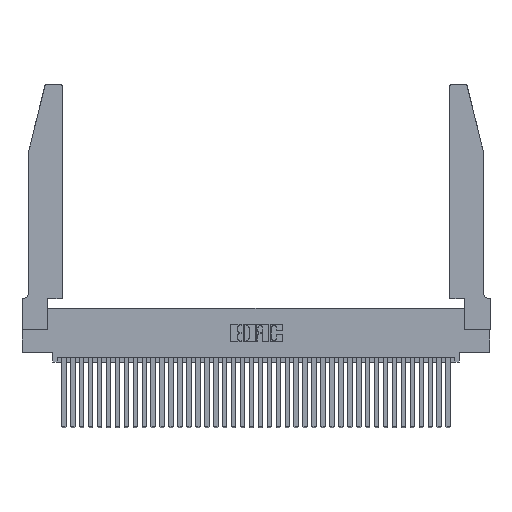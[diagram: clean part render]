
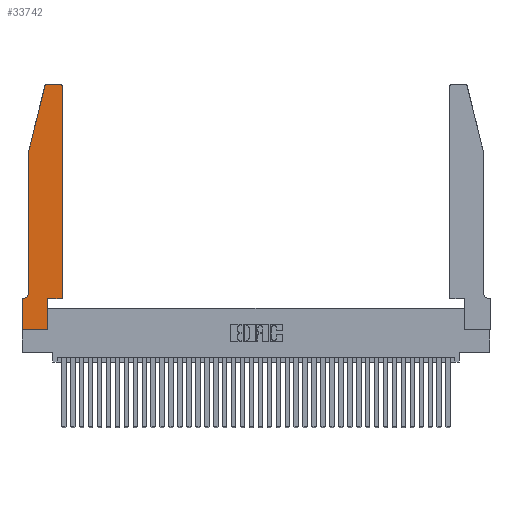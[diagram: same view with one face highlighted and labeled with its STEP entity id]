
A CAD part, top view. The second image highlights one B-rep face of the part: STEP entity #33742.
In plain terms, the highlighted planar face has unit normal (0, 0, 1).
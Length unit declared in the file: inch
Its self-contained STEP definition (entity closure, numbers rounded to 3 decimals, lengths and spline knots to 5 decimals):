
#1102 = EDGE_CURVE ( 'NONE', #10972, #13277, #33385, .T. ) ;
#1503 = VERTEX_POINT ( 'NONE', #20617 ) ;
#1673 = CARTESIAN_POINT ( 'NONE',  ( 0.0755, 2., 0.37 ) ) ;
#1690 = DIRECTION ( 'NONE',  ( 1., 0., 0. ) ) ;
#2762 = DIRECTION ( 'NONE',  ( 0., -1., 0. ) ) ;
#3133 = DIRECTION ( 'NONE',  ( 1., 0., 0. ) ) ;
#3369 = LINE ( 'NONE', #26260, #16984 ) ;
#3413 = LINE ( 'NONE', #1673, #31639 ) ;
#3737 = ORIENTED_EDGE ( 'NONE', *, *, #11222, .T. ) ;
#3932 = ORIENTED_EDGE ( 'NONE', *, *, #10514, .T. ) ;
#5132 = ORIENTED_EDGE ( 'NONE', *, *, #38542, .T. ) ;
#5758 = AXIS2_PLACEMENT_3D ( 'NONE', #37495, #10068, #19400 ) ;
#5767 = CARTESIAN_POINT ( 'NONE',  ( 0.4505, 0.35, 0.37 ) ) ;
#5779 = DIRECTION ( 'NONE',  ( 1., 0., 0. ) ) ;
#6118 = VERTEX_POINT ( 'NONE', #27946 ) ;
#7369 = CARTESIAN_POINT ( 'NONE',  ( 0.0755, 2., 0.37 ) ) ;
#7943 = ORIENTED_EDGE ( 'NONE', *, *, #11675, .T. ) ;
#8167 = EDGE_CURVE ( 'NONE', #6118, #37233, #38728, .T. ) ;
#8539 = CARTESIAN_POINT ( 'NONE',  ( 0., 0., 0.37 ) ) ;
#9168 = VECTOR ( 'NONE', #2762, 39.37008 ) ;
#9340 = AXIS2_PLACEMENT_3D ( 'NONE', #27116, #26991, #33083 ) ;
#9657 = DIRECTION ( 'NONE',  ( 0., 1., 0. ) ) ;
#10068 = DIRECTION ( 'NONE',  ( 0., 0., -1. ) ) ;
#10113 = ORIENTED_EDGE ( 'NONE', *, *, #28743, .T. ) ;
#10354 = VECTOR ( 'NONE', #3133, 39.37008 ) ;
#10514 = EDGE_CURVE ( 'NONE', #37233, #19504, #33564, .T. ) ;
#10587 = VERTEX_POINT ( 'NONE', #28307 ) ;
#10622 = CARTESIAN_POINT ( 'NONE',  ( 0.284, 2.72, 0.37 ) ) ;
#10972 = VERTEX_POINT ( 'NONE', #17748 ) ;
#11222 = EDGE_CURVE ( 'NONE', #36231, #1503, #25538, .T. ) ;
#11424 = PLANE ( 'NONE',  #25909 ) ;
#11675 = EDGE_CURVE ( 'NONE', #10587, #27237, #3369, .T. ) ;
#12286 = CARTESIAN_POINT ( 'NONE',  ( 0.0055, 0.35, 0.37 ) ) ;
#13109 = CARTESIAN_POINT ( 'NONE',  ( 0.0755, 0.35, 0.37 ) ) ;
#13259 = LINE ( 'NONE', #21642, #21733 ) ;
#13277 = VERTEX_POINT ( 'NONE', #37921 ) ;
#13508 = CIRCLE ( 'NONE', #5758, 0.07 ) ;
#13902 = EDGE_CURVE ( 'NONE', #13277, #36231, #13508, .T. ) ;
#15530 = ORIENTED_EDGE ( 'NONE', *, *, #8167, .T. ) ;
#16342 = DIRECTION ( 'NONE',  ( 1., 0., 0. ) ) ;
#16609 = DIRECTION ( 'NONE',  ( 0., 0., 1. ) ) ;
#16892 = ORIENTED_EDGE ( 'NONE', *, *, #26562, .T. ) ;
#16984 = VECTOR ( 'NONE', #26904, 39.37008 ) ;
#17439 = VECTOR ( 'NONE', #16342, 39.37008 ) ;
#17500 = VECTOR ( 'NONE', #9657, 39.37008 ) ;
#17505 = VECTOR ( 'NONE', #18923, 39.37008 ) ;
#17748 = CARTESIAN_POINT ( 'NONE',  ( 0.0755, 2., 0.37 ) ) ;
#18323 = LINE ( 'NONE', #5767, #10354 ) ;
#18704 = AXIS2_PLACEMENT_3D ( 'NONE', #10622, #16609, #1690 ) ;
#18923 = DIRECTION ( 'NONE',  ( -1., 0., 0. ) ) ;
#19398 = DIRECTION ( 'NONE',  ( -0.239, -0.971, 0. ) ) ;
#19400 = DIRECTION ( 'NONE',  ( -1., 0., 0. ) ) ;
#19466 = ORIENTED_EDGE ( 'NONE', *, *, #1102, .T. ) ;
#19504 = VERTEX_POINT ( 'NONE', #29045 ) ;
#19529 = CARTESIAN_POINT ( 'NONE',  ( 0., 0., 0.37 ) ) ;
#20617 = CARTESIAN_POINT ( 'NONE',  ( 0., 0.35, 0.37 ) ) ;
#20677 = EDGE_CURVE ( 'NONE', #27237, #36382, #22739, .T. ) ;
#21576 = EDGE_LOOP ( 'NONE', ( #7943, #35192, #33126, #19466, #24120, #3737, #33429, #15530, #3932, #16892, #10113, #5132 ) ) ;
#21642 = CARTESIAN_POINT ( 'NONE',  ( 0.4505, 0.35, 0.37 ) ) ;
#21733 = VECTOR ( 'NONE', #30726, 39.37008 ) ;
#22739 = CIRCLE ( 'NONE', #18704, 0.03 ) ;
#23288 = CARTESIAN_POINT ( 'NONE',  ( 0.2865, 0., 0.37 ) ) ;
#23658 = CARTESIAN_POINT ( 'NONE',  ( 0., 0.35, 0.37 ) ) ;
#24016 = CIRCLE ( 'NONE', #9340, 0.03 ) ;
#24120 = ORIENTED_EDGE ( 'NONE', *, *, #13902, .T. ) ;
#24608 = VERTEX_POINT ( 'NONE', #25740 ) ;
#24628 = CARTESIAN_POINT ( 'NONE',  ( 0.2865, 0.35, 0.37 ) ) ;
#24858 = CARTESIAN_POINT ( 'NONE',  ( 0.4505, 2.72, 0.37 ) ) ;
#25191 = EDGE_CURVE ( 'NONE', #36382, #10972, #3413, .T. ) ;
#25538 = LINE ( 'NONE', #13109, #17505 ) ;
#25740 = CARTESIAN_POINT ( 'NONE',  ( 0.4505, 0.35, 0.37 ) ) ;
#25909 = AXIS2_PLACEMENT_3D ( 'NONE', #23658, #32484, #5779 ) ;
#26260 = CARTESIAN_POINT ( 'NONE',  ( 0.2605, 2.75, 0.37 ) ) ;
#26562 = EDGE_CURVE ( 'NONE', #19504, #24608, #18323, .T. ) ;
#26904 = DIRECTION ( 'NONE',  ( -1., 0., 0. ) ) ;
#26991 = DIRECTION ( 'NONE',  ( 0., 0., 1. ) ) ;
#27116 = CARTESIAN_POINT ( 'NONE',  ( 0.4205, 2.72, 0.37 ) ) ;
#27237 = VERTEX_POINT ( 'NONE', #32966 ) ;
#27480 = LINE ( 'NONE', #8539, #9168 ) ;
#27946 = CARTESIAN_POINT ( 'NONE',  ( 0., 0., 0.37 ) ) ;
#28307 = CARTESIAN_POINT ( 'NONE',  ( 0.4205, 2.75, 0.37 ) ) ;
#28743 = EDGE_CURVE ( 'NONE', #24608, #33321, #13259, .T. ) ;
#29045 = CARTESIAN_POINT ( 'NONE',  ( 0.2865, 0.35, 0.37 ) ) ;
#30726 = DIRECTION ( 'NONE',  ( 0., 1., 0. ) ) ;
#31639 = VECTOR ( 'NONE', #19398, 39.37008 ) ;
#32484 = DIRECTION ( 'NONE',  ( 0., 0., 1. ) ) ;
#32966 = CARTESIAN_POINT ( 'NONE',  ( 0.284, 2.75, 0.37 ) ) ;
#33083 = DIRECTION ( 'NONE',  ( 1., 0., 0. ) ) ;
#33126 = ORIENTED_EDGE ( 'NONE', *, *, #25191, .T. ) ;
#33321 = VERTEX_POINT ( 'NONE', #24858 ) ;
#33385 = LINE ( 'NONE', #7369, #37194 ) ;
#33429 = ORIENTED_EDGE ( 'NONE', *, *, #33791, .T. ) ;
#33564 = LINE ( 'NONE', #24628, #17500 ) ;
#33643 = FACE_OUTER_BOUND ( 'NONE', #21576, .T. ) ;
#33742 = ADVANCED_FACE ( 'NONE', ( #33643 ), #11424, .T. ) ;
#33791 = EDGE_CURVE ( 'NONE', #1503, #6118, #27480, .T. ) ;
#35192 = ORIENTED_EDGE ( 'NONE', *, *, #20677, .T. ) ;
#36161 = DIRECTION ( 'NONE',  ( 0., -1., 0. ) ) ;
#36231 = VERTEX_POINT ( 'NONE', #12286 ) ;
#36382 = VERTEX_POINT ( 'NONE', #37624 ) ;
#37194 = VECTOR ( 'NONE', #36161, 39.37008 ) ;
#37233 = VERTEX_POINT ( 'NONE', #23288 ) ;
#37495 = CARTESIAN_POINT ( 'NONE',  ( 0.0055, 0.42, 0.37 ) ) ;
#37624 = CARTESIAN_POINT ( 'NONE',  ( 0.25487, 2.72718, 0.37 ) ) ;
#37921 = CARTESIAN_POINT ( 'NONE',  ( 0.0755, 0.42, 0.37 ) ) ;
#38542 = EDGE_CURVE ( 'NONE', #33321, #10587, #24016, .T. ) ;
#38728 = LINE ( 'NONE', #19529, #17439 ) ;
